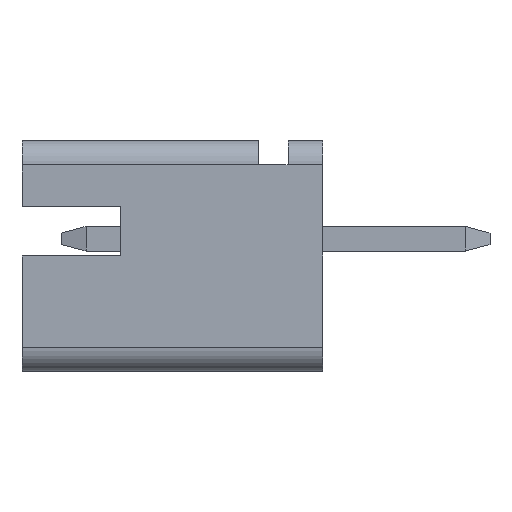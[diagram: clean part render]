
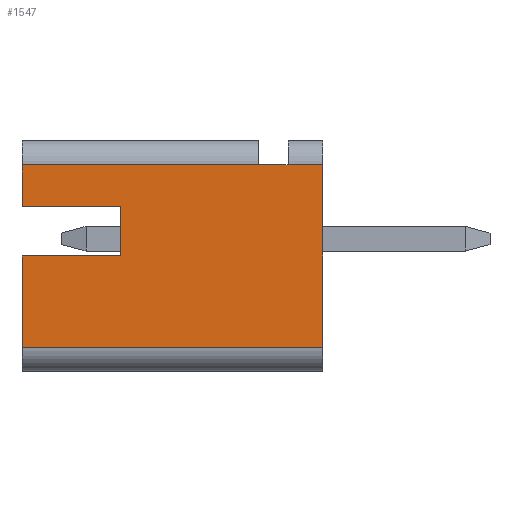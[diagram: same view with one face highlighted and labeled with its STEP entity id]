
A CAD part, left-side view. The second image highlights one B-rep face of the part: STEP entity #1547.
In plain terms, the highlighted planar face has unit normal (-1, 0, 0).
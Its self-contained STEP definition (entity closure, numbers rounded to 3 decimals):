
#54 = VECTOR ( 'NONE', #1815, 1000. ) ;
#99 = CARTESIAN_POINT ( 'NONE',  ( -2., 6.1, 1.5 ) ) ;
#210 = EDGE_CURVE ( 'NONE', #1359, #3742, #4002, .T. ) ;
#239 = EDGE_CURVE ( 'NONE', #1498, #2060, #1515, .T. ) ;
#260 = CARTESIAN_POINT ( 'NONE',  ( -2., 6.1, -2.2 ) ) ;
#275 = CARTESIAN_POINT ( 'NONE',  ( -2., 4.1, 0.65 ) ) ;
#331 = DIRECTION ( 'NONE',  ( 0., -1., 0. ) ) ;
#344 = LINE ( 'NONE', #1658, #708 ) ;
#348 = LINE ( 'NONE', #601, #4118 ) ;
#374 = ORIENTED_EDGE ( 'NONE', *, *, #4084, .F. ) ;
#375 = CARTESIAN_POINT ( 'NONE',  ( -2., 0., 1.5 ) ) ;
#450 = ORIENTED_EDGE ( 'NONE', *, *, #3024, .T. ) ;
#478 = AXIS2_PLACEMENT_3D ( 'NONE', #2231, #1856, #2878 ) ;
#490 = VERTEX_POINT ( 'NONE', #1480 ) ;
#514 = ORIENTED_EDGE ( 'NONE', *, *, #1721, .T. ) ;
#530 = CARTESIAN_POINT ( 'NONE',  ( -2., 0., 1.5 ) ) ;
#601 = CARTESIAN_POINT ( 'NONE',  ( -2., 0., 1.5 ) ) ;
#656 = ORIENTED_EDGE ( 'NONE', *, *, #2944, .F. ) ;
#667 = CARTESIAN_POINT ( 'NONE',  ( -2., 6.1, 2. ) ) ;
#678 = VERTEX_POINT ( 'NONE', #907 ) ;
#694 = CARTESIAN_POINT ( 'NONE',  ( -2., 6.1, 0.65 ) ) ;
#708 = VECTOR ( 'NONE', #2640, 1000. ) ;
#817 = ORIENTED_EDGE ( 'NONE', *, *, #3069, .F. ) ;
#862 = CARTESIAN_POINT ( 'NONE',  ( -2., 0., -2.2 ) ) ;
#907 = CARTESIAN_POINT ( 'NONE',  ( -2., 1.3, 1.5 ) ) ;
#919 = VECTOR ( 'NONE', #3739, 1000. ) ;
#955 = CARTESIAN_POINT ( 'NONE',  ( -2., 0.7, 1.5 ) ) ;
#973 = DIRECTION ( 'NONE',  ( 0., 1., 0. ) ) ;
#1097 = VECTOR ( 'NONE', #331, 1000. ) ;
#1184 = LINE ( 'NONE', #530, #3373 ) ;
#1235 = VERTEX_POINT ( 'NONE', #955 ) ;
#1247 = LINE ( 'NONE', #667, #1796 ) ;
#1305 = CARTESIAN_POINT ( 'NONE',  ( -2., 6.1, 0.65 ) ) ;
#1359 = VERTEX_POINT ( 'NONE', #2693 ) ;
#1480 = CARTESIAN_POINT ( 'NONE',  ( -2., 4.1, -0.35 ) ) ;
#1498 = VERTEX_POINT ( 'NONE', #375 ) ;
#1501 = ORIENTED_EDGE ( 'NONE', *, *, #3626, .F. ) ;
#1515 = LINE ( 'NONE', #3674, #3261 ) ;
#1547 = ADVANCED_FACE ( 'NONE', ( #3557 ), #1897, .F. ) ;
#1601 = DIRECTION ( 'NONE',  ( 0., 0., 1. ) ) ;
#1658 = CARTESIAN_POINT ( 'NONE',  ( -2., 0., -2.2 ) ) ;
#1702 = VERTEX_POINT ( 'NONE', #3262 ) ;
#1717 = CARTESIAN_POINT ( 'NONE',  ( -2., 1.3, 1.5 ) ) ;
#1721 = EDGE_CURVE ( 'NONE', #678, #2812, #348, .T. ) ;
#1796 = VECTOR ( 'NONE', #1601, 1000. ) ;
#1815 = DIRECTION ( 'NONE',  ( 0., 0., 1. ) ) ;
#1856 = DIRECTION ( 'NONE',  ( 1., 0., 0. ) ) ;
#1897 = PLANE ( 'NONE',  #478 ) ;
#1976 = DIRECTION ( 'NONE',  ( 0., 0., -1. ) ) ;
#1995 = EDGE_LOOP ( 'NONE', ( #2952, #450, #2216, #2753, #817, #514, #374, #2744, #656, #1501 ) ) ;
#2060 = VERTEX_POINT ( 'NONE', #862 ) ;
#2213 = DIRECTION ( 'NONE',  ( 0., 1., 0. ) ) ;
#2216 = ORIENTED_EDGE ( 'NONE', *, *, #239, .F. ) ;
#2231 = CARTESIAN_POINT ( 'NONE',  ( -2., 0., 0. ) ) ;
#2254 = EDGE_CURVE ( 'NONE', #3970, #1702, #2522, .T. ) ;
#2330 = EDGE_CURVE ( 'NONE', #1498, #1235, #1184, .T. ) ;
#2522 = LINE ( 'NONE', #3517, #54 ) ;
#2628 = LINE ( 'NONE', #2947, #1097 ) ;
#2640 = DIRECTION ( 'NONE',  ( 0., -1., 0. ) ) ;
#2680 = LINE ( 'NONE', #1717, #919 ) ;
#2693 = CARTESIAN_POINT ( 'NONE',  ( -2., 4.1, 0.65 ) ) ;
#2744 = ORIENTED_EDGE ( 'NONE', *, *, #210, .F. ) ;
#2745 = VECTOR ( 'NONE', #3300, 1000. ) ;
#2753 = ORIENTED_EDGE ( 'NONE', *, *, #2330, .T. ) ;
#2812 = VERTEX_POINT ( 'NONE', #99 ) ;
#2878 = DIRECTION ( 'NONE',  ( 0., 0., -1. ) ) ;
#2903 = DIRECTION ( 'NONE',  ( 0., 1., 0. ) ) ;
#2944 = EDGE_CURVE ( 'NONE', #490, #1359, #3614, .T. ) ;
#2947 = CARTESIAN_POINT ( 'NONE',  ( -2., 6.1, -0.35 ) ) ;
#2952 = ORIENTED_EDGE ( 'NONE', *, *, #2254, .F. ) ;
#3024 = EDGE_CURVE ( 'NONE', #3970, #2060, #344, .T. ) ;
#3069 = EDGE_CURVE ( 'NONE', #678, #1235, #2680, .T. ) ;
#3261 = VECTOR ( 'NONE', #1976, 1000. ) ;
#3262 = CARTESIAN_POINT ( 'NONE',  ( -2., 6.1, -0.35 ) ) ;
#3300 = DIRECTION ( 'NONE',  ( 0., 0., 1. ) ) ;
#3373 = VECTOR ( 'NONE', #2213, 1000. ) ;
#3517 = CARTESIAN_POINT ( 'NONE',  ( -2., 6.1, -0.35 ) ) ;
#3557 = FACE_OUTER_BOUND ( 'NONE', #1995, .T. ) ;
#3614 = LINE ( 'NONE', #275, #2745 ) ;
#3626 = EDGE_CURVE ( 'NONE', #1702, #490, #2628, .T. ) ;
#3674 = CARTESIAN_POINT ( 'NONE',  ( -2., 0., 2. ) ) ;
#3739 = DIRECTION ( 'NONE',  ( 0., -1., 0. ) ) ;
#3742 = VERTEX_POINT ( 'NONE', #694 ) ;
#3747 = VECTOR ( 'NONE', #2903, 1000. ) ;
#3970 = VERTEX_POINT ( 'NONE', #260 ) ;
#4002 = LINE ( 'NONE', #1305, #3747 ) ;
#4084 = EDGE_CURVE ( 'NONE', #3742, #2812, #1247, .T. ) ;
#4118 = VECTOR ( 'NONE', #973, 1000. ) ;
